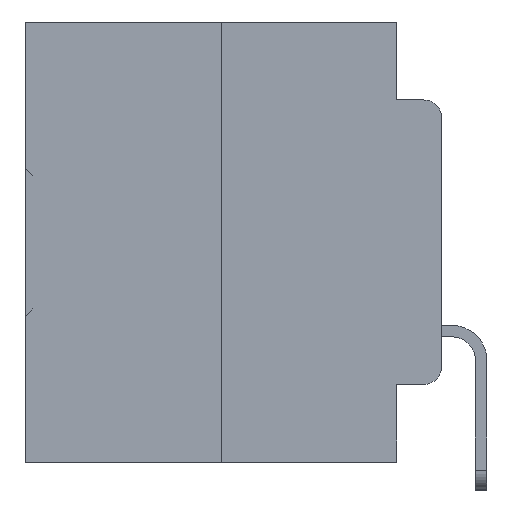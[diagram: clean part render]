
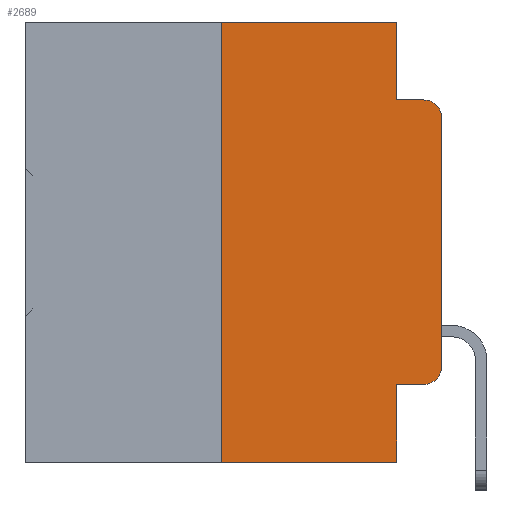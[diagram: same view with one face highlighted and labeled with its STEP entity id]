
A CAD part, left-side view. The second image highlights one B-rep face of the part: STEP entity #2689.
In plain terms, the highlighted planar face has unit normal (-1, 0, 0).
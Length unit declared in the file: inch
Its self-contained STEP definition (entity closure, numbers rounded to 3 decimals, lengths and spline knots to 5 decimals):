
#544 = VECTOR ( 'NONE', #26015, 39.37008 ) ;
#975 = VERTEX_POINT ( 'NONE', #28765 ) ;
#1354 = VERTEX_POINT ( 'NONE', #30363 ) ;
#1673 = CARTESIAN_POINT ( 'NONE',  ( 0., 0., -0.3915 ) ) ;
#2689 = ADVANCED_FACE ( 'NONE', ( #23246 ), #27957, .F. ) ;
#2743 = EDGE_CURVE ( 'NONE', #7642, #21785, #22386, .T. ) ;
#3629 = EDGE_CURVE ( 'NONE', #34233, #20372, #17231, .T. ) ;
#3670 = EDGE_CURVE ( 'NONE', #21785, #8232, #22739, .T. ) ;
#3674 = CARTESIAN_POINT ( 'NONE',  ( 0., 0.02, -0.1085 ) ) ;
#3692 = AXIS2_PLACEMENT_3D ( 'NONE', #3674, #23682, #6661 ) ;
#4714 = LINE ( 'NONE', #22549, #11751 ) ;
#4935 = VERTEX_POINT ( 'NONE', #1673 ) ;
#5460 = LINE ( 'NONE', #6459, #19960 ) ;
#5669 = ORIENTED_EDGE ( 'NONE', *, *, #3670, .F. ) ;
#6459 = CARTESIAN_POINT ( 'NONE',  ( 0., 0., 0. ) ) ;
#6661 = DIRECTION ( 'NONE',  ( 0., 0., -1. ) ) ;
#7057 = ORIENTED_EDGE ( 'NONE', *, *, #3629, .T. ) ;
#7642 = VERTEX_POINT ( 'NONE', #19818 ) ;
#8067 = EDGE_LOOP ( 'NONE', ( #36361, #31012, #18440, #27267, #5669, #23493, #18878, #13129, #7057, #31040 ) ) ;
#8232 = VERTEX_POINT ( 'NONE', #32637 ) ;
#8244 = DIRECTION ( 'NONE',  ( -1., 0., 0. ) ) ;
#8546 = VECTOR ( 'NONE', #12715, 39.37008 ) ;
#11751 = VECTOR ( 'NONE', #19861, 39.37008 ) ;
#11753 = DIRECTION ( 'NONE',  ( 0., -1., 0. ) ) ;
#12150 = VECTOR ( 'NONE', #11753, 39.37008 ) ;
#12715 = DIRECTION ( 'NONE',  ( 0., -1., 0. ) ) ;
#12757 = EDGE_CURVE ( 'NONE', #8232, #1354, #4714, .T. ) ;
#13129 = ORIENTED_EDGE ( 'NONE', *, *, #26355, .F. ) ;
#13551 = VECTOR ( 'NONE', #25130, 39.37008 ) ;
#14320 = CIRCLE ( 'NONE', #3692, 0.02 ) ;
#14372 = DIRECTION ( 'NONE',  ( 1., 0., 0. ) ) ;
#14510 = CARTESIAN_POINT ( 'NONE',  ( 0., 0., -0.1085 ) ) ;
#14742 = CARTESIAN_POINT ( 'NONE',  ( 0., 0.25, 0. ) ) ;
#15134 = CARTESIAN_POINT ( 'NONE',  ( 0., 0.02, -0.4115 ) ) ;
#15597 = CARTESIAN_POINT ( 'NONE',  ( 0., 0.473, 0. ) ) ;
#16363 = LINE ( 'NONE', #23430, #544 ) ;
#17231 = LINE ( 'NONE', #18438, #8546 ) ;
#17463 = CIRCLE ( 'NONE', #18177, 0.02 ) ;
#17507 = CARTESIAN_POINT ( 'NONE',  ( 0., 0.051, -0.0885 ) ) ;
#18177 = AXIS2_PLACEMENT_3D ( 'NONE', #25103, #8244, #27813 ) ;
#18205 = DIRECTION ( 'NONE',  ( 0., 0., 1. ) ) ;
#18438 = CARTESIAN_POINT ( 'NONE',  ( 0., 0.051, -0.4115 ) ) ;
#18440 = ORIENTED_EDGE ( 'NONE', *, *, #22066, .F. ) ;
#18878 = ORIENTED_EDGE ( 'NONE', *, *, #33542, .T. ) ;
#19719 = AXIS2_PLACEMENT_3D ( 'NONE', #19858, #14372, #33281 ) ;
#19818 = CARTESIAN_POINT ( 'NONE',  ( 0., 0.25, -0.5 ) ) ;
#19858 = CARTESIAN_POINT ( 'NONE',  ( 0., 0.473, 0. ) ) ;
#19861 = DIRECTION ( 'NONE',  ( 0., 0., -1. ) ) ;
#19960 = VECTOR ( 'NONE', #18205, 39.37008 ) ;
#20349 = VERTEX_POINT ( 'NONE', #14510 ) ;
#20372 = VERTEX_POINT ( 'NONE', #15134 ) ;
#21760 = VERTEX_POINT ( 'NONE', #27180 ) ;
#21785 = VERTEX_POINT ( 'NONE', #29858 ) ;
#22066 = EDGE_CURVE ( 'NONE', #1354, #21760, #33878, .T. ) ;
#22386 = LINE ( 'NONE', #14742, #28705 ) ;
#22549 = CARTESIAN_POINT ( 'NONE',  ( 0., 0.051, 0. ) ) ;
#22739 = LINE ( 'NONE', #15597, #36055 ) ;
#23246 = FACE_OUTER_BOUND ( 'NONE', #8067, .T. ) ;
#23430 = CARTESIAN_POINT ( 'NONE',  ( 0., 0.473, -0.5 ) ) ;
#23493 = ORIENTED_EDGE ( 'NONE', *, *, #2743, .F. ) ;
#23682 = DIRECTION ( 'NONE',  ( -1., 0., 0. ) ) ;
#23728 = CARTESIAN_POINT ( 'NONE',  ( 0., 0.051, -0.4115 ) ) ;
#23943 = DIRECTION ( 'NONE',  ( 0., -1., 0. ) ) ;
#25103 = CARTESIAN_POINT ( 'NONE',  ( 0., 0.02, -0.3915 ) ) ;
#25130 = DIRECTION ( 'NONE',  ( 0., 0., -1. ) ) ;
#26015 = DIRECTION ( 'NONE',  ( 0., -1., 0. ) ) ;
#26355 = EDGE_CURVE ( 'NONE', #34233, #975, #28096, .T. ) ;
#27180 = CARTESIAN_POINT ( 'NONE',  ( 0., 0.02, -0.0885 ) ) ;
#27267 = ORIENTED_EDGE ( 'NONE', *, *, #12757, .F. ) ;
#27813 = DIRECTION ( 'NONE',  ( 0., 0., -1. ) ) ;
#27957 = PLANE ( 'NONE',  #19719 ) ;
#28096 = LINE ( 'NONE', #33045, #13551 ) ;
#28602 = EDGE_CURVE ( 'NONE', #4935, #20349, #5460, .T. ) ;
#28705 = VECTOR ( 'NONE', #30973, 39.37008 ) ;
#28765 = CARTESIAN_POINT ( 'NONE',  ( 0., 0.051, -0.5 ) ) ;
#28928 = EDGE_CURVE ( 'NONE', #20372, #4935, #17463, .T. ) ;
#29273 = EDGE_CURVE ( 'NONE', #20349, #21760, #14320, .T. ) ;
#29858 = CARTESIAN_POINT ( 'NONE',  ( 0., 0.25, 0. ) ) ;
#30363 = CARTESIAN_POINT ( 'NONE',  ( 0., 0.051, -0.0885 ) ) ;
#30973 = DIRECTION ( 'NONE',  ( 0., 0., 1. ) ) ;
#31012 = ORIENTED_EDGE ( 'NONE', *, *, #29273, .T. ) ;
#31040 = ORIENTED_EDGE ( 'NONE', *, *, #28928, .T. ) ;
#32637 = CARTESIAN_POINT ( 'NONE',  ( 0., 0.051, 0. ) ) ;
#33045 = CARTESIAN_POINT ( 'NONE',  ( 0., 0.051, 0. ) ) ;
#33281 = DIRECTION ( 'NONE',  ( 0., 0., -1. ) ) ;
#33542 = EDGE_CURVE ( 'NONE', #7642, #975, #16363, .T. ) ;
#33878 = LINE ( 'NONE', #17507, #12150 ) ;
#34233 = VERTEX_POINT ( 'NONE', #23728 ) ;
#36055 = VECTOR ( 'NONE', #23943, 39.37008 ) ;
#36361 = ORIENTED_EDGE ( 'NONE', *, *, #28602, .T. ) ;
